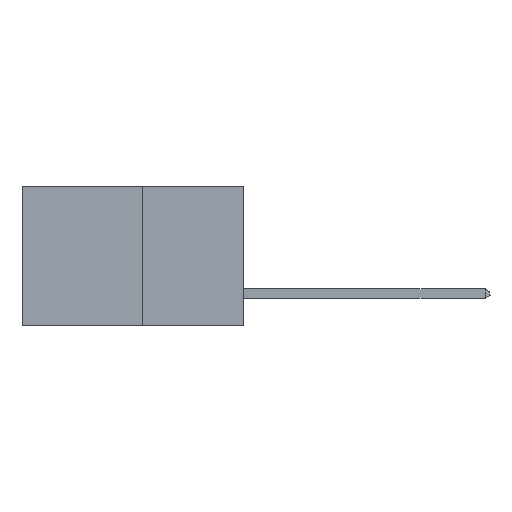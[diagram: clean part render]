
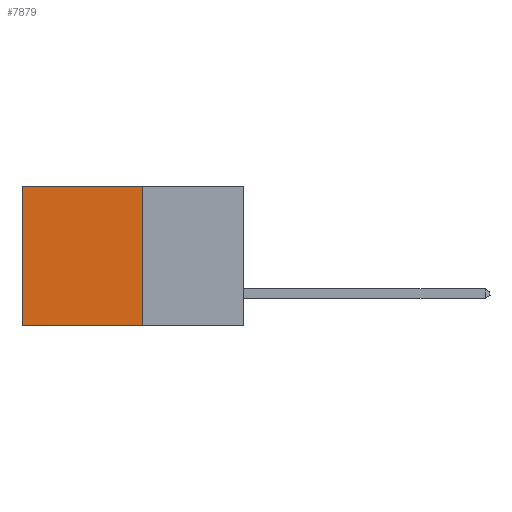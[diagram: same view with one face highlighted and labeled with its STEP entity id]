
A CAD part, left-side view. The second image highlights one B-rep face of the part: STEP entity #7879.
In plain terms, the highlighted planar face has unit normal (-1, 0, 0).
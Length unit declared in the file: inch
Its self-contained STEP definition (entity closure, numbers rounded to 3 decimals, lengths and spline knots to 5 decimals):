
#646 = LINE ( 'NONE', #7495, #8656 ) ;
#766 = CARTESIAN_POINT ( 'NONE',  ( 0.277, 0.27, 0. ) ) ;
#881 = EDGE_CURVE ( 'NONE', #7575, #4765, #12055, .T. ) ;
#981 = EDGE_CURVE ( 'NONE', #11054, #3358, #9146, .T. ) ;
#1668 = ORIENTED_EDGE ( 'NONE', *, *, #981, .F. ) ;
#1982 = EDGE_CURVE ( 'NONE', #4765, #3358, #646, .T. ) ;
#1987 = EDGE_CURVE ( 'NONE', #7575, #11054, #6054, .T. ) ;
#2063 = ORIENTED_EDGE ( 'NONE', *, *, #1987, .F. ) ;
#3358 = VERTEX_POINT ( 'NONE', #7624 ) ;
#3534 = PLANE ( 'NONE',  #12011 ) ;
#3592 = CARTESIAN_POINT ( 'NONE',  ( 0.277, 0.27, -0.37 ) ) ;
#3667 = FACE_OUTER_BOUND ( 'NONE', #3696, .T. ) ;
#3696 = EDGE_LOOP ( 'NONE', ( #9115, #1668, #2063, #7735 ) ) ;
#3933 = CARTESIAN_POINT ( 'NONE',  ( 0.277, 0.59, 0. ) ) ;
#4733 = DIRECTION ( 'NONE',  ( 0., 0., -1. ) ) ;
#4765 = VERTEX_POINT ( 'NONE', #3933 ) ;
#4865 = CARTESIAN_POINT ( 'NONE',  ( 0.277, 0.27, -0.37 ) ) ;
#5921 = DIRECTION ( 'NONE',  ( 0., 0., -1. ) ) ;
#6054 = LINE ( 'NONE', #8389, #10874 ) ;
#7012 = VECTOR ( 'NONE', #9607, 39.37008 ) ;
#7495 = CARTESIAN_POINT ( 'NONE',  ( 0.277, 0.59, -0.37 ) ) ;
#7575 = VERTEX_POINT ( 'NONE', #766 ) ;
#7624 = CARTESIAN_POINT ( 'NONE',  ( 0.277, 0.59, -0.37 ) ) ;
#7735 = ORIENTED_EDGE ( 'NONE', *, *, #881, .T. ) ;
#7879 = ADVANCED_FACE ( 'NONE', ( #3667 ), #3534, .F. ) ;
#8059 = CARTESIAN_POINT ( 'NONE',  ( 0.277, 0.27, -0.37 ) ) ;
#8361 = CARTESIAN_POINT ( 'NONE',  ( 0.277, 0.27, 0. ) ) ;
#8389 = CARTESIAN_POINT ( 'NONE',  ( 0.277, 0.27, -0.37 ) ) ;
#8535 = DIRECTION ( 'NONE',  ( 0., 0., -1. ) ) ;
#8656 = VECTOR ( 'NONE', #8535, 39.37008 ) ;
#9115 = ORIENTED_EDGE ( 'NONE', *, *, #1982, .T. ) ;
#9146 = LINE ( 'NONE', #4865, #11058 ) ;
#9607 = DIRECTION ( 'NONE',  ( 0., 1., 0. ) ) ;
#10583 = DIRECTION ( 'NONE',  ( 1., 0., 0. ) ) ;
#10874 = VECTOR ( 'NONE', #5921, 39.37008 ) ;
#11054 = VERTEX_POINT ( 'NONE', #8059 ) ;
#11058 = VECTOR ( 'NONE', #12881, 39.37008 ) ;
#12011 = AXIS2_PLACEMENT_3D ( 'NONE', #3592, #10583, #4733 ) ;
#12055 = LINE ( 'NONE', #8361, #7012 ) ;
#12881 = DIRECTION ( 'NONE',  ( 0., 1., 0. ) ) ;
